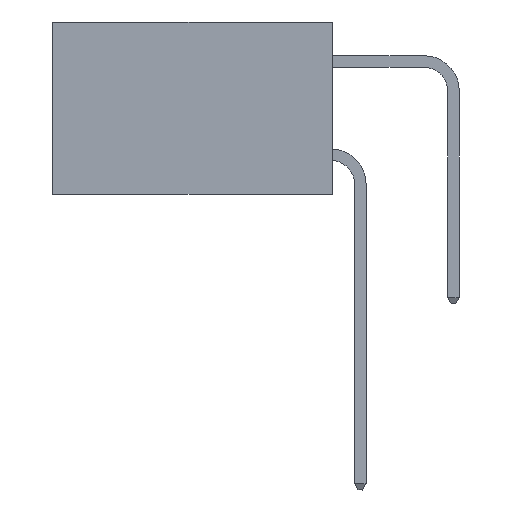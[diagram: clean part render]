
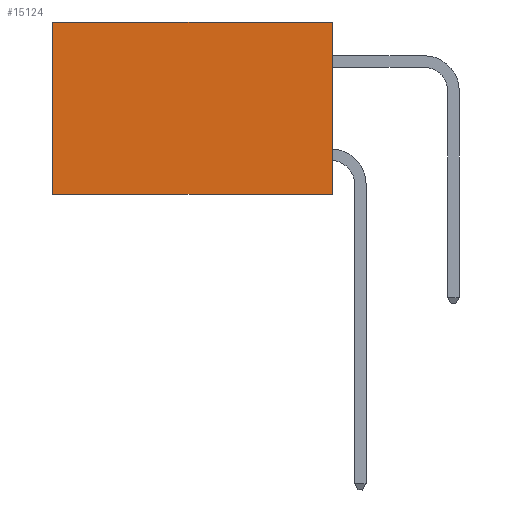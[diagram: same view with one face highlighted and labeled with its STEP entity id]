
A CAD part, left-side view. The second image highlights one B-rep face of the part: STEP entity #15124.
In plain terms, the highlighted planar face has unit normal (-1, 0, 0).
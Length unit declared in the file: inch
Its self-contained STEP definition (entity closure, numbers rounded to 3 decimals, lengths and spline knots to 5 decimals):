
#1251 = EDGE_CURVE ( 'NONE', #12824, #7309, #20467, .T. ) ;
#1712 = DIRECTION ( 'NONE',  ( 0., 1., 0. ) ) ;
#1859 = DIRECTION ( 'NONE',  ( 0., 0., -1. ) ) ;
#1945 = DIRECTION ( 'NONE',  ( 0., 0., -1. ) ) ;
#1988 = VECTOR ( 'NONE', #1712, 39.37008 ) ;
#3823 = VERTEX_POINT ( 'NONE', #4776 ) ;
#3861 = ORIENTED_EDGE ( 'NONE', *, *, #1251, .T. ) ;
#4050 = CARTESIAN_POINT ( 'NONE',  ( 0.2615, 0.6, -0.37 ) ) ;
#4776 = CARTESIAN_POINT ( 'NONE',  ( 0.2615, 0., -0.37 ) ) ;
#6004 = VECTOR ( 'NONE', #14268, 39.37008 ) ;
#6362 = LINE ( 'NONE', #18220, #1988 ) ;
#6555 = VECTOR ( 'NONE', #1859, 39.37008 ) ;
#7309 = VERTEX_POINT ( 'NONE', #4050 ) ;
#7388 = CARTESIAN_POINT ( 'NONE',  ( 0.2615, 0., -0.37 ) ) ;
#8566 = CARTESIAN_POINT ( 'NONE',  ( 0.2615, 0.6, 0. ) ) ;
#10356 = PLANE ( 'NONE',  #15845 ) ;
#10455 = CARTESIAN_POINT ( 'NONE',  ( 0.2615, 0., 0. ) ) ;
#12371 = CARTESIAN_POINT ( 'NONE',  ( 0.2615, 0., -0.37 ) ) ;
#12390 = EDGE_CURVE ( 'NONE', #20819, #3823, #15376, .T. ) ;
#12628 = EDGE_CURVE ( 'NONE', #20819, #12824, #6362, .T. ) ;
#12824 = VERTEX_POINT ( 'NONE', #8566 ) ;
#14268 = DIRECTION ( 'NONE',  ( 0., 1., 0. ) ) ;
#15124 = ADVANCED_FACE ( 'NONE', ( #18784 ), #10356, .F. ) ;
#15376 = LINE ( 'NONE', #12371, #6555 ) ;
#15845 = AXIS2_PLACEMENT_3D ( 'NONE', #17122, #17333, #1945 ) ;
#16690 = ORIENTED_EDGE ( 'NONE', *, *, #12390, .F. ) ;
#17122 = CARTESIAN_POINT ( 'NONE',  ( 0.2615, 0., -0.37 ) ) ;
#17144 = DIRECTION ( 'NONE',  ( 0., 0., -1. ) ) ;
#17333 = DIRECTION ( 'NONE',  ( 1., 0., 0. ) ) ;
#17363 = LINE ( 'NONE', #7388, #6004 ) ;
#17416 = ORIENTED_EDGE ( 'NONE', *, *, #21812, .F. ) ;
#18220 = CARTESIAN_POINT ( 'NONE',  ( 0.2615, 0., 0. ) ) ;
#18268 = ORIENTED_EDGE ( 'NONE', *, *, #12628, .T. ) ;
#18784 = FACE_OUTER_BOUND ( 'NONE', #20461, .T. ) ;
#18863 = VECTOR ( 'NONE', #17144, 39.37008 ) ;
#20461 = EDGE_LOOP ( 'NONE', ( #3861, #17416, #16690, #18268 ) ) ;
#20467 = LINE ( 'NONE', #20583, #18863 ) ;
#20583 = CARTESIAN_POINT ( 'NONE',  ( 0.2615, 0.6, -0.37 ) ) ;
#20819 = VERTEX_POINT ( 'NONE', #10455 ) ;
#21812 = EDGE_CURVE ( 'NONE', #3823, #7309, #17363, .T. ) ;
